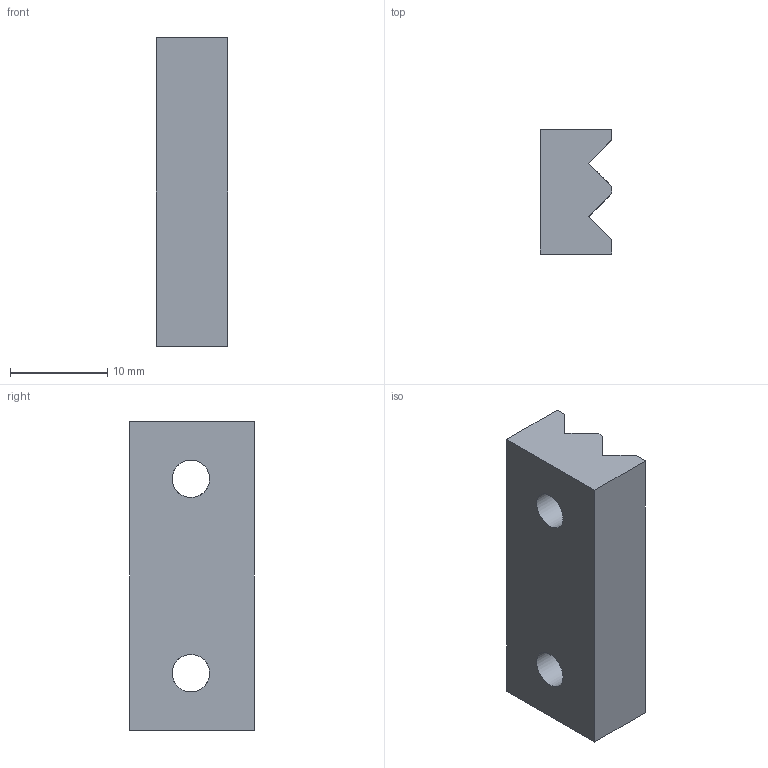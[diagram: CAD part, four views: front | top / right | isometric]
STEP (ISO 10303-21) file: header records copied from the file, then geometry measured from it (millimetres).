
FILE_DESCRIPTION(/* description */ ('STEP AP214'),/* implementation_level */ '2;1');
FILE_NAME(/* name */ 'Slat.stp',/* time_stamp */ '2019-08-10T22:58:17-05:00',/* author */ ('johne'),/* organization */ (''),/* preprocessor_version */ 'ST-DEVELOPER v16.13',/* originating_system */ 'Autodesk Inventor 2018',/* authorisation */ '');
FILE_SCHEMA (('AUTOMOTIVE_DESIGN { 1 0 10303 214 3 1 1 }'));
Length unit declared in the file: inch
Products named in the file (1): Slat
Bounding box: 7.4 x 12.83 x 31.75 mm (x, y, z)
Volume: 2488.5 mm3; surface area: 1681.1 mm2
Topology: 1 solids, 1 shells, 16 faces, 48 edges, 32 vertices
Faces by surface type: plane 14, cylinder 2
Full cylindrical faces by diameter (mm): 3.858 x2
Entity records: 563 total; most frequent: CARTESIAN_POINT 91, ORIENTED_EDGE 88, DIRECTION 88, EDGE_CURVE 44, LINE 34, VECTOR 34, VERTEX_POINT 30, AXIS2_PLACEMENT_3D 27
